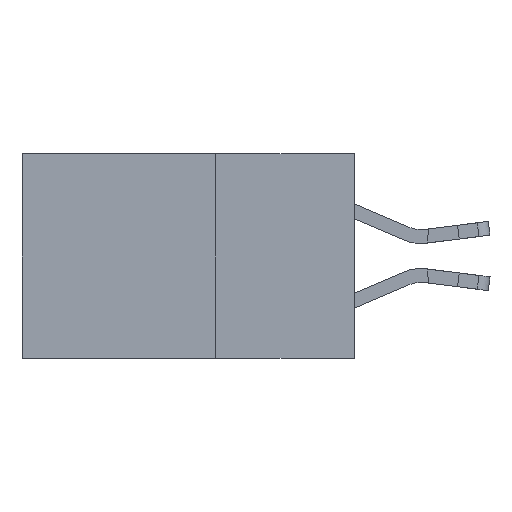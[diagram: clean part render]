
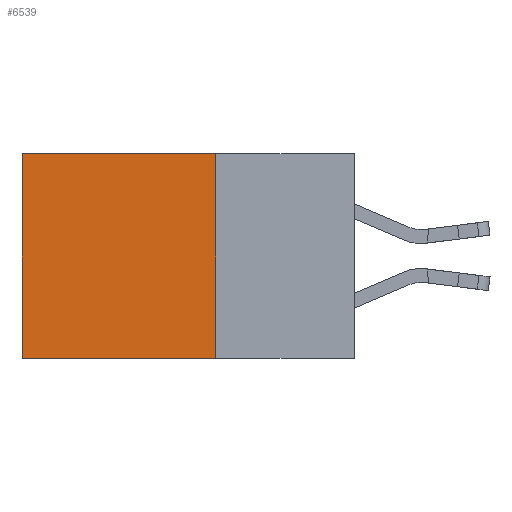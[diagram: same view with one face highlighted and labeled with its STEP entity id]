
A CAD part, left-side view. The second image highlights one B-rep face of the part: STEP entity #6539.
In plain terms, the highlighted planar face has unit normal (-1, 0, 0).
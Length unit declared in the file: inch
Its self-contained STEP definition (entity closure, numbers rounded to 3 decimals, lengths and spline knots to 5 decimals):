
#391 = EDGE_CURVE ( 'NONE', #6636, #14013, #7535, .T. ) ;
#482 = CARTESIAN_POINT ( 'NONE',  ( 0.2615, 0.6, -0.37 ) ) ;
#570 = DIRECTION ( 'NONE',  ( 0., 0., -1. ) ) ;
#914 = EDGE_LOOP ( 'NONE', ( #9582, #3645, #13985, #1510 ) ) ;
#1510 = ORIENTED_EDGE ( 'NONE', *, *, #391, .T. ) ;
#2299 = FACE_OUTER_BOUND ( 'NONE', #914, .T. ) ;
#2354 = VECTOR ( 'NONE', #570, 39.37008 ) ;
#2683 = VERTEX_POINT ( 'NONE', #2866 ) ;
#2695 = LINE ( 'NONE', #482, #2354 ) ;
#2866 = CARTESIAN_POINT ( 'NONE',  ( 0.2615, 0.6, -0.37 ) ) ;
#3645 = ORIENTED_EDGE ( 'NONE', *, *, #5556, .F. ) ;
#4147 = CARTESIAN_POINT ( 'NONE',  ( 0.2615, 0.25, 0. ) ) ;
#4390 = VERTEX_POINT ( 'NONE', #6381 ) ;
#5472 = EDGE_CURVE ( 'NONE', #14013, #2683, #2695, .T. ) ;
#5556 = EDGE_CURVE ( 'NONE', #4390, #2683, #12579, .T. ) ;
#6381 = CARTESIAN_POINT ( 'NONE',  ( 0.2615, 0.25, -0.37 ) ) ;
#6402 = DIRECTION ( 'NONE',  ( 0., 1., 0. ) ) ;
#6539 = ADVANCED_FACE ( 'NONE', ( #2299 ), #9294, .F. ) ;
#6556 = CARTESIAN_POINT ( 'NONE',  ( 0.2615, 0.6, 0. ) ) ;
#6636 = VERTEX_POINT ( 'NONE', #10068 ) ;
#7535 = LINE ( 'NONE', #4147, #13006 ) ;
#7939 = CARTESIAN_POINT ( 'NONE',  ( 0.2615, 0.25, -0.37 ) ) ;
#8102 = DIRECTION ( 'NONE',  ( 0., 1., 0. ) ) ;
#8489 = DIRECTION ( 'NONE',  ( 0., 0., -1. ) ) ;
#8513 = DIRECTION ( 'NONE',  ( 1., 0., 0. ) ) ;
#8517 = CARTESIAN_POINT ( 'NONE',  ( 0.2615, 0.25, -0.37 ) ) ;
#9294 = PLANE ( 'NONE',  #10823 ) ;
#9582 = ORIENTED_EDGE ( 'NONE', *, *, #5472, .T. ) ;
#9651 = LINE ( 'NONE', #10173, #12192 ) ;
#9684 = VECTOR ( 'NONE', #8102, 39.37008 ) ;
#10068 = CARTESIAN_POINT ( 'NONE',  ( 0.2615, 0.25, 0. ) ) ;
#10173 = CARTESIAN_POINT ( 'NONE',  ( 0.2615, 0.25, -0.37 ) ) ;
#10176 = DIRECTION ( 'NONE',  ( 0., 0., -1. ) ) ;
#10823 = AXIS2_PLACEMENT_3D ( 'NONE', #8517, #8513, #8489 ) ;
#12192 = VECTOR ( 'NONE', #10176, 39.37008 ) ;
#12579 = LINE ( 'NONE', #7939, #9684 ) ;
#13006 = VECTOR ( 'NONE', #6402, 39.37008 ) ;
#13490 = EDGE_CURVE ( 'NONE', #6636, #4390, #9651, .T. ) ;
#13985 = ORIENTED_EDGE ( 'NONE', *, *, #13490, .F. ) ;
#14013 = VERTEX_POINT ( 'NONE', #6556 ) ;
